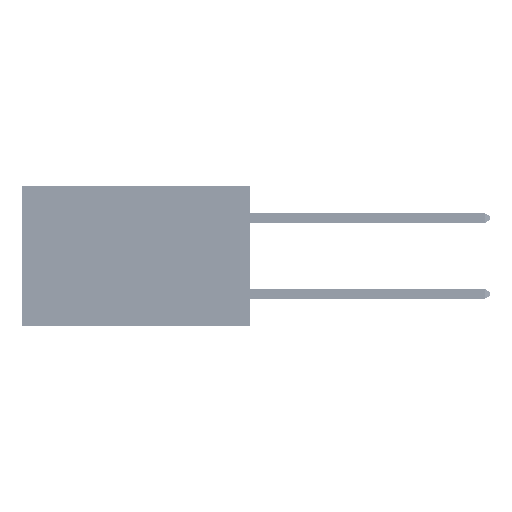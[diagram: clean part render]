
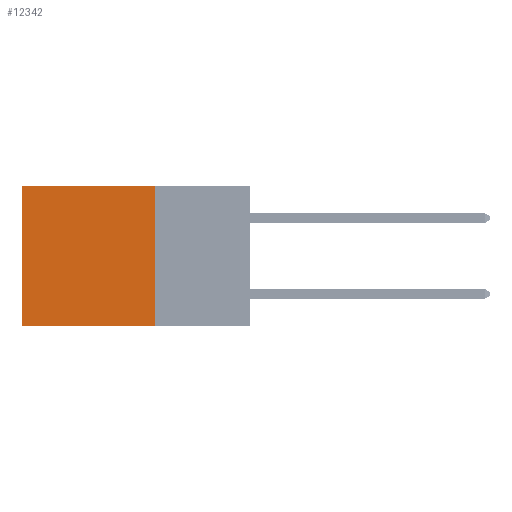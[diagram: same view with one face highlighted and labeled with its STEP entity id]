
A CAD part, left-side view. The second image highlights one B-rep face of the part: STEP entity #12342.
In plain terms, the highlighted planar face has unit normal (-1, 0, 0).
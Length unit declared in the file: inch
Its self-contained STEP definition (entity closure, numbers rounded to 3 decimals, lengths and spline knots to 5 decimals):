
#491 = PLANE ( 'NONE',  #4743 ) ;
#980 = DIRECTION ( 'NONE',  ( 0., 0., -1. ) ) ;
#4209 = FACE_OUTER_BOUND ( 'NONE', #14321, .T. ) ;
#4391 = VECTOR ( 'NONE', #11486, 39.37008 ) ;
#4743 = AXIS2_PLACEMENT_3D ( 'NONE', #12159, #42429, #980 ) ;
#4890 = ORIENTED_EDGE ( 'NONE', *, *, #30044, .T. ) ;
#6704 = CARTESIAN_POINT ( 'NONE',  ( 0.2875, 0.6, -0.37 ) ) ;
#9621 = LINE ( 'NONE', #28747, #29766 ) ;
#11056 = DIRECTION ( 'NONE',  ( 0., 1., 0. ) ) ;
#11486 = DIRECTION ( 'NONE',  ( 0., 1., 0. ) ) ;
#12159 = CARTESIAN_POINT ( 'NONE',  ( 0.2875, 0.25, 0. ) ) ;
#12197 = EDGE_CURVE ( 'NONE', #22232, #27627, #48171, .T. ) ;
#12342 = ADVANCED_FACE ( 'NONE', ( #4209 ), #491, .F. ) ;
#14284 = LINE ( 'NONE', #44071, #4391 ) ;
#14321 = EDGE_LOOP ( 'NONE', ( #4890, #31855, #16903, #14625 ) ) ;
#14625 = ORIENTED_EDGE ( 'NONE', *, *, #18030, .T. ) ;
#16903 = ORIENTED_EDGE ( 'NONE', *, *, #12197, .F. ) ;
#18030 = EDGE_CURVE ( 'NONE', #22232, #22242, #45566, .T. ) ;
#22232 = VERTEX_POINT ( 'NONE', #46087 ) ;
#22242 = VERTEX_POINT ( 'NONE', #42122 ) ;
#24507 = DIRECTION ( 'NONE',  ( 0., 0., -1. ) ) ;
#25363 = VECTOR ( 'NONE', #36765, 39.37008 ) ;
#25805 = VECTOR ( 'NONE', #11056, 39.37008 ) ;
#26977 = VERTEX_POINT ( 'NONE', #6704 ) ;
#27627 = VERTEX_POINT ( 'NONE', #34362 ) ;
#28747 = CARTESIAN_POINT ( 'NONE',  ( 0.2875, 0.6, 0. ) ) ;
#29325 = CARTESIAN_POINT ( 'NONE',  ( 0.2875, 0.25, 0. ) ) ;
#29766 = VECTOR ( 'NONE', #24507, 39.37008 ) ;
#30044 = EDGE_CURVE ( 'NONE', #22242, #26977, #9621, .T. ) ;
#30596 = EDGE_CURVE ( 'NONE', #27627, #26977, #14284, .T. ) ;
#31855 = ORIENTED_EDGE ( 'NONE', *, *, #30596, .F. ) ;
#33415 = CARTESIAN_POINT ( 'NONE',  ( 0.2875, 0.25, 0. ) ) ;
#34362 = CARTESIAN_POINT ( 'NONE',  ( 0.2875, 0.25, -0.37 ) ) ;
#36765 = DIRECTION ( 'NONE',  ( 0., 0., -1. ) ) ;
#42122 = CARTESIAN_POINT ( 'NONE',  ( 0.2875, 0.6, 0. ) ) ;
#42429 = DIRECTION ( 'NONE',  ( 1., 0., 0. ) ) ;
#44071 = CARTESIAN_POINT ( 'NONE',  ( 0.2875, 0.25, -0.37 ) ) ;
#45566 = LINE ( 'NONE', #33415, #25805 ) ;
#46087 = CARTESIAN_POINT ( 'NONE',  ( 0.2875, 0.25, 0. ) ) ;
#48171 = LINE ( 'NONE', #29325, #25363 ) ;
